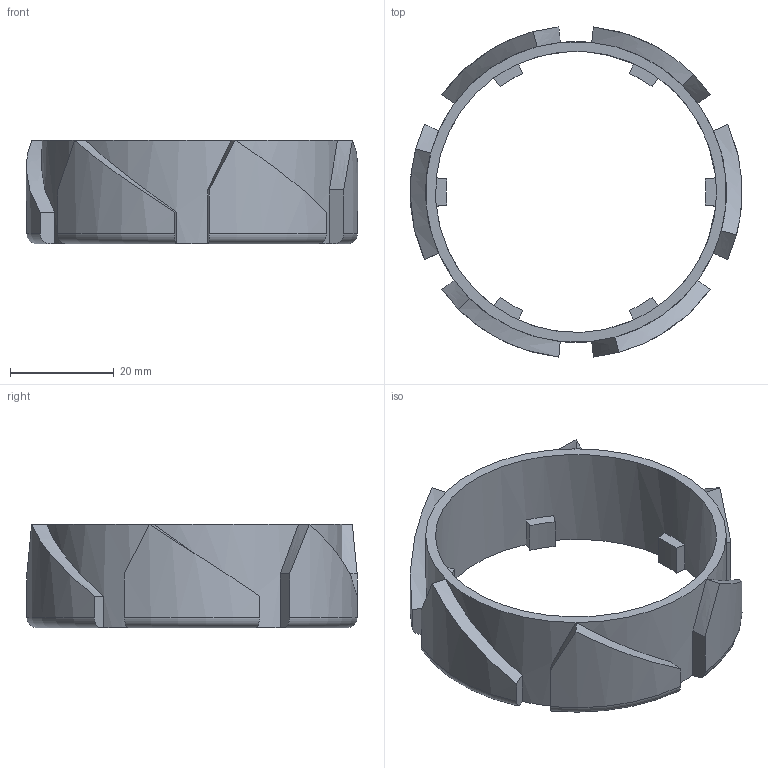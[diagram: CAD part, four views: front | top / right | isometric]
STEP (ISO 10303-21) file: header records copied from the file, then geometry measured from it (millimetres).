
FILE_DESCRIPTION((''),'2;1');
FILE_NAME('PM522NYLONRearIndexRing2.stp','2015-10-01T18:19:36',('JamesRPatrick'),(''),'Autodesk Inventor 2012','Autodesk Inventor 2012','');
FILE_SCHEMA(('AUTOMOTIVE_DESIGN { 1 0 10303 214 1 1 1 1 }'));
Length unit declared in the file: millimetre
Products named in the file (1): PM522NYLONRearIndexRing2
Bounding box: 63.97 x 63.65 x 20 mm (x, y, z)
Volume: 13131.4 mm3; surface area: 9430.9 mm2
Topology: 1 solids, 1 shells, 69 faces, 189 edges, 122 vertices
Faces by surface type: plane 32, cylinder 19, bspline 12, torus 6
Full cylindrical faces by diameter (mm): 54.2 x1
Entity records: 2420 total; most frequent: CARTESIAN_POINT 702, ORIENTED_EDGE 374, DIRECTION 328, EDGE_CURVE 187, VERTEX_POINT 121, AXIS2_PLACEMENT_3D 119, VECTOR 90, LINE 90
